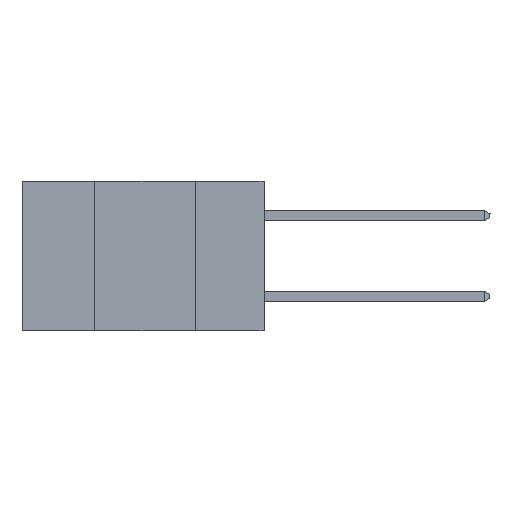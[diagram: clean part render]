
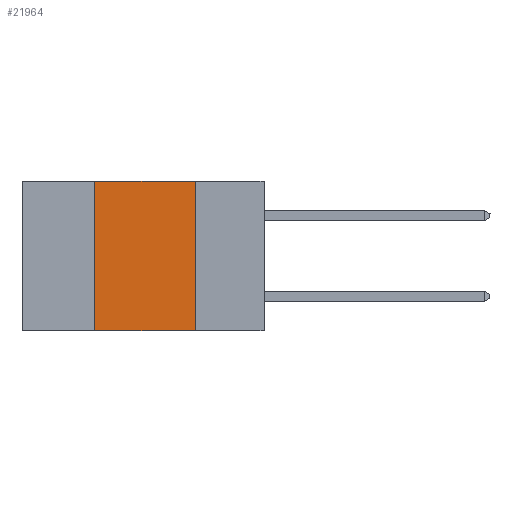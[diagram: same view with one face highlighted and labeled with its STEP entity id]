
A CAD part, left-side view. The second image highlights one B-rep face of the part: STEP entity #21964.
In plain terms, the highlighted planar face has unit normal (-1, 0, 0).
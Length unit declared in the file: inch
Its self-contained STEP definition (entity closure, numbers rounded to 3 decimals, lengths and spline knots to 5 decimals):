
#268 = DIRECTION ( 'NONE',  ( 1., 0., 0. ) ) ;
#1991 = ORIENTED_EDGE ( 'NONE', *, *, #11111, .T. ) ;
#2226 = LINE ( 'NONE', #4942, #21840 ) ;
#2481 = EDGE_CURVE ( 'NONE', #19138, #17933, #2226, .T. ) ;
#2620 = VERTEX_POINT ( 'NONE', #32315 ) ;
#4665 = LINE ( 'NONE', #31548, #32255 ) ;
#4711 = EDGE_LOOP ( 'NONE', ( #27941, #27349, #28103, #1991 ) ) ;
#4942 = CARTESIAN_POINT ( 'NONE',  ( 0., 0.17, 0. ) ) ;
#5335 = CARTESIAN_POINT ( 'NONE',  ( 0., 0.42, 0. ) ) ;
#5890 = AXIS2_PLACEMENT_3D ( 'NONE', #30587, #268, #18307 ) ;
#7062 = DIRECTION ( 'NONE',  ( 0., 0., -1. ) ) ;
#7643 = EDGE_CURVE ( 'NONE', #2620, #12113, #24520, .T. ) ;
#7924 = DIRECTION ( 'NONE',  ( 0., 0., 1. ) ) ;
#8919 = DIRECTION ( 'NONE',  ( 0., -1., 0. ) ) ;
#10746 = CARTESIAN_POINT ( 'NONE',  ( 0., 0.17, 0. ) ) ;
#11082 = VECTOR ( 'NONE', #7924, 39.37008 ) ;
#11111 = EDGE_CURVE ( 'NONE', #2620, #17933, #4665, .T. ) ;
#12113 = VERTEX_POINT ( 'NONE', #30618 ) ;
#12748 = DIRECTION ( 'NONE',  ( 0., -1., 0. ) ) ;
#16731 = FACE_OUTER_BOUND ( 'NONE', #4711, .T. ) ;
#17933 = VERTEX_POINT ( 'NONE', #21285 ) ;
#18307 = DIRECTION ( 'NONE',  ( 0., 0., -1. ) ) ;
#19138 = VERTEX_POINT ( 'NONE', #10746 ) ;
#20353 = CARTESIAN_POINT ( 'NONE',  ( 0., 0.6, 0. ) ) ;
#20515 = EDGE_CURVE ( 'NONE', #12113, #19138, #23433, .T. ) ;
#21285 = CARTESIAN_POINT ( 'NONE',  ( 0., 0.17, -0.37 ) ) ;
#21840 = VECTOR ( 'NONE', #7062, 39.37008 ) ;
#21964 = ADVANCED_FACE ( 'NONE', ( #16731 ), #28075, .F. ) ;
#23433 = LINE ( 'NONE', #20353, #29965 ) ;
#24520 = LINE ( 'NONE', #5335, #11082 ) ;
#27349 = ORIENTED_EDGE ( 'NONE', *, *, #20515, .F. ) ;
#27941 = ORIENTED_EDGE ( 'NONE', *, *, #2481, .F. ) ;
#28075 = PLANE ( 'NONE',  #5890 ) ;
#28103 = ORIENTED_EDGE ( 'NONE', *, *, #7643, .F. ) ;
#29965 = VECTOR ( 'NONE', #12748, 39.37008 ) ;
#30587 = CARTESIAN_POINT ( 'NONE',  ( 0., 0.6, 0. ) ) ;
#30618 = CARTESIAN_POINT ( 'NONE',  ( 0., 0.42, 0. ) ) ;
#31548 = CARTESIAN_POINT ( 'NONE',  ( 0., 0.6, -0.37 ) ) ;
#32255 = VECTOR ( 'NONE', #8919, 39.37008 ) ;
#32315 = CARTESIAN_POINT ( 'NONE',  ( 0., 0.42, -0.37 ) ) ;
